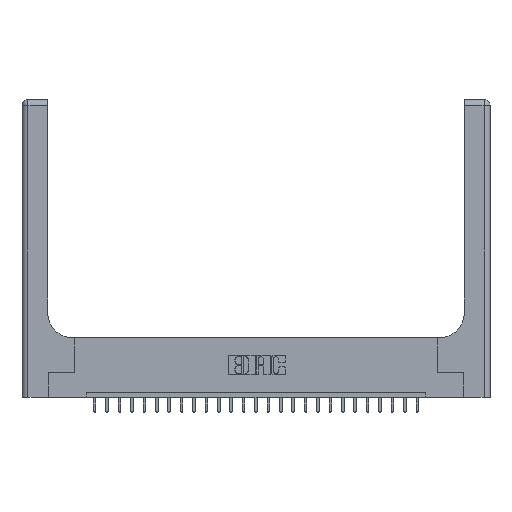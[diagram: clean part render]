
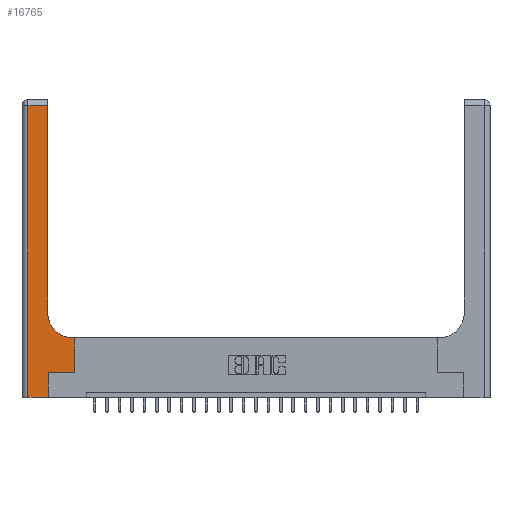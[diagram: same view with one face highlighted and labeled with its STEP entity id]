
A CAD part, top view. The second image highlights one B-rep face of the part: STEP entity #16765.
In plain terms, the highlighted planar face has unit normal (0, 0, 1).
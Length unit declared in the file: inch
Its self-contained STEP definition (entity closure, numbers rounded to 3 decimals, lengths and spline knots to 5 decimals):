
#731 = LINE ( 'NONE', #14346, #21805 ) ;
#751 = DIRECTION ( 'NONE',  ( -1., 0., 0. ) ) ;
#920 = AXIS2_PLACEMENT_3D ( 'NONE', #19810, #20170, #2896 ) ;
#1382 = VECTOR ( 'NONE', #23081, 39.37008 ) ;
#1614 = VECTOR ( 'NONE', #751, 39.37008 ) ;
#2428 = FACE_OUTER_BOUND ( 'NONE', #11630, .T. ) ;
#2616 = DIRECTION ( 'NONE',  ( 1., 0., 0. ) ) ;
#2896 = DIRECTION ( 'NONE',  ( 1., 0., 0. ) ) ;
#3209 = EDGE_CURVE ( 'NONE', #10553, #13629, #12144, .T. ) ;
#3647 = ORIENTED_EDGE ( 'NONE', *, *, #10818, .T. ) ;
#3767 = CARTESIAN_POINT ( 'NONE',  ( 0.528, 0.6, 0.37 ) ) ;
#4397 = VECTOR ( 'NONE', #15717, 39.37008 ) ;
#4625 = CARTESIAN_POINT ( 'NONE',  ( 0.06, 3., 0.37 ) ) ;
#5205 = CARTESIAN_POINT ( 'NONE',  ( 0.26, 0.85, 0.37 ) ) ;
#5646 = AXIS2_PLACEMENT_3D ( 'NONE', #15785, #21325, #6389 ) ;
#5915 = EDGE_CURVE ( 'NONE', #9343, #13218, #8033, .T. ) ;
#5959 = CARTESIAN_POINT ( 'NONE',  ( 0.265, 0.25, 0.37 ) ) ;
#6389 = DIRECTION ( 'NONE',  ( -1., 0., 0. ) ) ;
#6437 = CIRCLE ( 'NONE', #920, 0.25 ) ;
#6639 = LINE ( 'NONE', #14316, #15917 ) ;
#6669 = DIRECTION ( 'NONE',  ( 0., 1., 0. ) ) ;
#6806 = LINE ( 'NONE', #23840, #16120 ) ;
#7640 = VECTOR ( 'NONE', #2616, 39.37008 ) ;
#7823 = LINE ( 'NONE', #5959, #7640 ) ;
#8033 = LINE ( 'NONE', #9652, #1382 ) ;
#8732 = EDGE_CURVE ( 'NONE', #13218, #13798, #17700, .T. ) ;
#9032 = ORIENTED_EDGE ( 'NONE', *, *, #15975, .T. ) ;
#9343 = VERTEX_POINT ( 'NONE', #21857 ) ;
#9402 = VECTOR ( 'NONE', #12037, 39.37008 ) ;
#9652 = CARTESIAN_POINT ( 'NONE',  ( 0., 2.94, 0.37 ) ) ;
#10027 = ORIENTED_EDGE ( 'NONE', *, *, #5915, .T. ) ;
#10120 = PLANE ( 'NONE',  #5646 ) ;
#10463 = CARTESIAN_POINT ( 'NONE',  ( 0.265, 0.25, 0.37 ) ) ;
#10553 = VERTEX_POINT ( 'NONE', #15112 ) ;
#10818 = EDGE_CURVE ( 'NONE', #20132, #13434, #6806, .T. ) ;
#11216 = ORIENTED_EDGE ( 'NONE', *, *, #8732, .T. ) ;
#11630 = EDGE_LOOP ( 'NONE', ( #9032, #10027, #11216, #17150, #3647, #14903, #16578, #15922, #18006 ) ) ;
#11753 = CARTESIAN_POINT ( 'NONE',  ( 0.51, 0.6, 0.37 ) ) ;
#12037 = DIRECTION ( 'NONE',  ( 0., -1., 0. ) ) ;
#12144 = LINE ( 'NONE', #12266, #4397 ) ;
#12266 = CARTESIAN_POINT ( 'NONE',  ( 0.528, 0.25, 0.37 ) ) ;
#13218 = VERTEX_POINT ( 'NONE', #19575 ) ;
#13434 = VERTEX_POINT ( 'NONE', #10463 ) ;
#13629 = VERTEX_POINT ( 'NONE', #3767 ) ;
#13798 = VERTEX_POINT ( 'NONE', #16114 ) ;
#14202 = EDGE_CURVE ( 'NONE', #13629, #23250, #21863, .T. ) ;
#14316 = CARTESIAN_POINT ( 'NONE',  ( 0., 0., 0.37 ) ) ;
#14346 = CARTESIAN_POINT ( 'NONE',  ( 0.26, 3., 0.37 ) ) ;
#14365 = DIRECTION ( 'NONE',  ( 0., 1., 0. ) ) ;
#14385 = CARTESIAN_POINT ( 'NONE',  ( 0.265, 0., 0.37 ) ) ;
#14903 = ORIENTED_EDGE ( 'NONE', *, *, #22810, .T. ) ;
#15112 = CARTESIAN_POINT ( 'NONE',  ( 0.528, 0.25, 0.37 ) ) ;
#15717 = DIRECTION ( 'NONE',  ( 0., 1., 0. ) ) ;
#15785 = CARTESIAN_POINT ( 'NONE',  ( 0., 3., 0.37 ) ) ;
#15917 = VECTOR ( 'NONE', #23418, 39.37008 ) ;
#15922 = ORIENTED_EDGE ( 'NONE', *, *, #14202, .T. ) ;
#15975 = EDGE_CURVE ( 'NONE', #21876, #9343, #731, .T. ) ;
#16114 = CARTESIAN_POINT ( 'NONE',  ( 0.06, 0., 0.37 ) ) ;
#16120 = VECTOR ( 'NONE', #14365, 39.37008 ) ;
#16578 = ORIENTED_EDGE ( 'NONE', *, *, #3209, .T. ) ;
#16765 = ADVANCED_FACE ( 'NONE', ( #2428 ), #10120, .F. ) ;
#16879 = EDGE_CURVE ( 'NONE', #13798, #20132, #6639, .T. ) ;
#17150 = ORIENTED_EDGE ( 'NONE', *, *, #16879, .T. ) ;
#17700 = LINE ( 'NONE', #4625, #9402 ) ;
#18006 = ORIENTED_EDGE ( 'NONE', *, *, #18489, .T. ) ;
#18489 = EDGE_CURVE ( 'NONE', #23250, #21876, #6437, .T. ) ;
#19575 = CARTESIAN_POINT ( 'NONE',  ( 0.06, 2.94, 0.37 ) ) ;
#19638 = CARTESIAN_POINT ( 'NONE',  ( 0.26, 0.6, 0.37 ) ) ;
#19810 = CARTESIAN_POINT ( 'NONE',  ( 0.51, 0.85, 0.37 ) ) ;
#20132 = VERTEX_POINT ( 'NONE', #14385 ) ;
#20170 = DIRECTION ( 'NONE',  ( 0., 0., -1. ) ) ;
#21325 = DIRECTION ( 'NONE',  ( 0., 0., -1. ) ) ;
#21805 = VECTOR ( 'NONE', #6669, 39.37008 ) ;
#21857 = CARTESIAN_POINT ( 'NONE',  ( 0.26, 2.94, 0.37 ) ) ;
#21863 = LINE ( 'NONE', #19638, #1614 ) ;
#21876 = VERTEX_POINT ( 'NONE', #5205 ) ;
#22810 = EDGE_CURVE ( 'NONE', #13434, #10553, #7823, .T. ) ;
#23081 = DIRECTION ( 'NONE',  ( -1., 0., 0. ) ) ;
#23250 = VERTEX_POINT ( 'NONE', #11753 ) ;
#23418 = DIRECTION ( 'NONE',  ( 1., 0., 0. ) ) ;
#23840 = CARTESIAN_POINT ( 'NONE',  ( 0.265, 0., 0.37 ) ) ;
